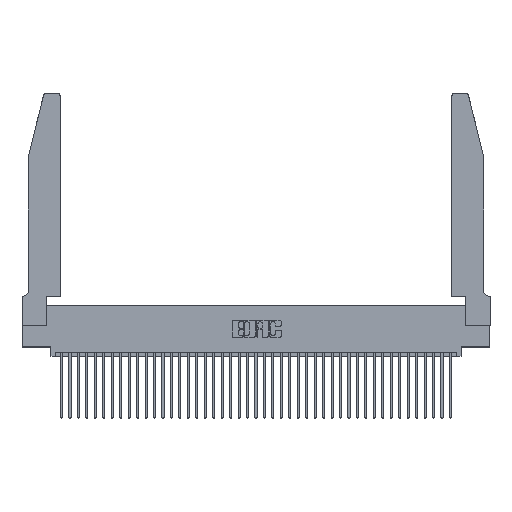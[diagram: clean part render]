
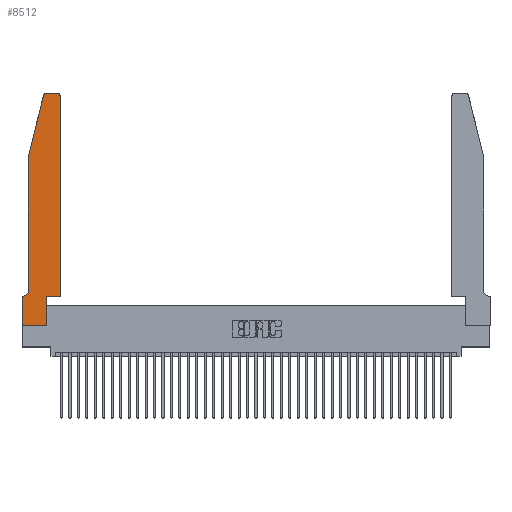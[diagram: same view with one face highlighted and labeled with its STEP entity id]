
A CAD part, top view. The second image highlights one B-rep face of the part: STEP entity #8512.
In plain terms, the highlighted planar face has unit normal (0, 0, 1).
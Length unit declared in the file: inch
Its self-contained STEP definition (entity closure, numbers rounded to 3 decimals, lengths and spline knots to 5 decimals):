
#678 = CARTESIAN_POINT ( 'NONE',  ( 0.0755, 0.35, 0.37 ) ) ;
#826 = CARTESIAN_POINT ( 'NONE',  ( 0.2865, 0.35, 0.37 ) ) ;
#832 = DIRECTION ( 'NONE',  ( 0., 0., -1. ) ) ;
#1188 = CARTESIAN_POINT ( 'NONE',  ( 0., 0., 0.37 ) ) ;
#1258 = CARTESIAN_POINT ( 'NONE',  ( 0.4505, 2.72, 0.37 ) ) ;
#1440 = AXIS2_PLACEMENT_3D ( 'NONE', #15298, #37526, #18527 ) ;
#1489 = VERTEX_POINT ( 'NONE', #26710 ) ;
#1978 = PLANE ( 'NONE',  #31422 ) ;
#2135 = CARTESIAN_POINT ( 'NONE',  ( 0., 0., 0.37 ) ) ;
#2276 = DIRECTION ( 'NONE',  ( -1., 0., 0. ) ) ;
#2727 = CARTESIAN_POINT ( 'NONE',  ( 0.4505, 0.35, 0.37 ) ) ;
#2892 = EDGE_CURVE ( 'NONE', #30835, #19793, #9939, .T. ) ;
#3472 = VERTEX_POINT ( 'NONE', #5498 ) ;
#3788 = ORIENTED_EDGE ( 'NONE', *, *, #40106, .T. ) ;
#4532 = CARTESIAN_POINT ( 'NONE',  ( 0.0755, 2., 0.37 ) ) ;
#5012 = AXIS2_PLACEMENT_3D ( 'NONE', #15292, #37517, #18522 ) ;
#5312 = LINE ( 'NONE', #4532, #30710 ) ;
#5498 = CARTESIAN_POINT ( 'NONE',  ( 0., 0.35, 0.37 ) ) ;
#5663 = DIRECTION ( 'NONE',  ( 0., -1., 0. ) ) ;
#6434 = CARTESIAN_POINT ( 'NONE',  ( 0.0055, 0.35, 0.37 ) ) ;
#6936 = CARTESIAN_POINT ( 'NONE',  ( 0., 0., 0.37 ) ) ;
#8348 = DIRECTION ( 'NONE',  ( 0., 0., 1. ) ) ;
#8512 = ADVANCED_FACE ( 'NONE', ( #18031 ), #1978, .T. ) ;
#8735 = VECTOR ( 'NONE', #26225, 39.37008 ) ;
#9711 = LINE ( 'NONE', #10306, #8735 ) ;
#9939 = LINE ( 'NONE', #2135, #10926 ) ;
#10101 = DIRECTION ( 'NONE',  ( 0., -1., 0. ) ) ;
#10306 = CARTESIAN_POINT ( 'NONE',  ( 0.4505, 0.35, 0.37 ) ) ;
#10403 = CIRCLE ( 'NONE', #15994, 0.07 ) ;
#10580 = EDGE_CURVE ( 'NONE', #26769, #32802, #10403, .T. ) ;
#10926 = VECTOR ( 'NONE', #24395, 39.37008 ) ;
#12018 = CARTESIAN_POINT ( 'NONE',  ( 0.2865, 0., 0.37 ) ) ;
#13012 = ORIENTED_EDGE ( 'NONE', *, *, #10580, .T. ) ;
#13527 = LINE ( 'NONE', #6936, #36921 ) ;
#14370 = ORIENTED_EDGE ( 'NONE', *, *, #40673, .T. ) ;
#14925 = EDGE_CURVE ( 'NONE', #25619, #15075, #20654, .T. ) ;
#15075 = VERTEX_POINT ( 'NONE', #37005 ) ;
#15106 = CARTESIAN_POINT ( 'NONE',  ( 0.0755, 2., 0.37 ) ) ;
#15292 = CARTESIAN_POINT ( 'NONE',  ( 0.284, 2.72, 0.37 ) ) ;
#15298 = CARTESIAN_POINT ( 'NONE',  ( 0.4205, 2.72, 0.37 ) ) ;
#15994 = AXIS2_PLACEMENT_3D ( 'NONE', #19891, #832, #23103 ) ;
#16298 = ORIENTED_EDGE ( 'NONE', *, *, #28432, .T. ) ;
#16540 = DIRECTION ( 'NONE',  ( -1., 0., 0. ) ) ;
#17356 = ORIENTED_EDGE ( 'NONE', *, *, #30061, .T. ) ;
#17877 = LINE ( 'NONE', #32700, #25348 ) ;
#18031 = FACE_OUTER_BOUND ( 'NONE', #25419, .T. ) ;
#18522 = DIRECTION ( 'NONE',  ( 1., 0., 0. ) ) ;
#18527 = DIRECTION ( 'NONE',  ( 1., 0., 0. ) ) ;
#18738 = ORIENTED_EDGE ( 'NONE', *, *, #28729, .T. ) ;
#19155 = LINE ( 'NONE', #678, #26623 ) ;
#19793 = VERTEX_POINT ( 'NONE', #12018 ) ;
#19803 = VECTOR ( 'NONE', #5663, 39.37008 ) ;
#19891 = CARTESIAN_POINT ( 'NONE',  ( 0.0055, 0.42, 0.37 ) ) ;
#20654 = CIRCLE ( 'NONE', #1440, 0.03 ) ;
#20676 = CIRCLE ( 'NONE', #5012, 0.03 ) ;
#20862 = VECTOR ( 'NONE', #2276, 39.37008 ) ;
#21792 = DIRECTION ( 'NONE',  ( 0., 1., 0. ) ) ;
#21812 = LINE ( 'NONE', #15106, #19803 ) ;
#21869 = LINE ( 'NONE', #33970, #20862 ) ;
#23038 = VERTEX_POINT ( 'NONE', #33370 ) ;
#23103 = DIRECTION ( 'NONE',  ( -1., 0., 0. ) ) ;
#23373 = ORIENTED_EDGE ( 'NONE', *, *, #2892, .T. ) ;
#24395 = DIRECTION ( 'NONE',  ( 1., 0., 0. ) ) ;
#25348 = VECTOR ( 'NONE', #35876, 39.37008 ) ;
#25419 = EDGE_LOOP ( 'NONE', ( #36100, #16298, #3788, #39818, #13012, #18738, #17356, #23373, #39348, #14370, #31836, #27286 ) ) ;
#25512 = EDGE_CURVE ( 'NONE', #19793, #30121, #17877, .T. ) ;
#25619 = VERTEX_POINT ( 'NONE', #1258 ) ;
#26225 = DIRECTION ( 'NONE',  ( 1., 0., 0. ) ) ;
#26614 = CARTESIAN_POINT ( 'NONE',  ( 0.25487, 2.72718, 0.37 ) ) ;
#26623 = VECTOR ( 'NONE', #16540, 39.37008 ) ;
#26710 = CARTESIAN_POINT ( 'NONE',  ( 0.4505, 0.35, 0.37 ) ) ;
#26769 = VERTEX_POINT ( 'NONE', #35604 ) ;
#27130 = EDGE_CURVE ( 'NONE', #23038, #26769, #21812, .T. ) ;
#27286 = ORIENTED_EDGE ( 'NONE', *, *, #14925, .T. ) ;
#27428 = CARTESIAN_POINT ( 'NONE',  ( 0., 0.35, 0.37 ) ) ;
#28214 = VECTOR ( 'NONE', #21792, 39.37008 ) ;
#28432 = EDGE_CURVE ( 'NONE', #33786, #38752, #20676, .T. ) ;
#28729 = EDGE_CURVE ( 'NONE', #32802, #3472, #19155, .T. ) ;
#30061 = EDGE_CURVE ( 'NONE', #3472, #30835, #13527, .T. ) ;
#30121 = VERTEX_POINT ( 'NONE', #826 ) ;
#30608 = DIRECTION ( 'NONE',  ( 1., 0., 0. ) ) ;
#30710 = VECTOR ( 'NONE', #39517, 39.37008 ) ;
#30835 = VERTEX_POINT ( 'NONE', #1188 ) ;
#31422 = AXIS2_PLACEMENT_3D ( 'NONE', #27428, #8348, #30608 ) ;
#31836 = ORIENTED_EDGE ( 'NONE', *, *, #40400, .T. ) ;
#32700 = CARTESIAN_POINT ( 'NONE',  ( 0.2865, 0.35, 0.37 ) ) ;
#32802 = VERTEX_POINT ( 'NONE', #6434 ) ;
#33370 = CARTESIAN_POINT ( 'NONE',  ( 0.0755, 2., 0.37 ) ) ;
#33786 = VERTEX_POINT ( 'NONE', #37351 ) ;
#33970 = CARTESIAN_POINT ( 'NONE',  ( 0.2605, 2.75, 0.37 ) ) ;
#35604 = CARTESIAN_POINT ( 'NONE',  ( 0.0755, 0.42, 0.37 ) ) ;
#35654 = LINE ( 'NONE', #2727, #28214 ) ;
#35876 = DIRECTION ( 'NONE',  ( 0., 1., 0. ) ) ;
#36100 = ORIENTED_EDGE ( 'NONE', *, *, #39022, .T. ) ;
#36921 = VECTOR ( 'NONE', #10101, 39.37008 ) ;
#37005 = CARTESIAN_POINT ( 'NONE',  ( 0.4205, 2.75, 0.37 ) ) ;
#37351 = CARTESIAN_POINT ( 'NONE',  ( 0.284, 2.75, 0.37 ) ) ;
#37517 = DIRECTION ( 'NONE',  ( 0., 0., 1. ) ) ;
#37526 = DIRECTION ( 'NONE',  ( 0., 0., 1. ) ) ;
#38752 = VERTEX_POINT ( 'NONE', #26614 ) ;
#39022 = EDGE_CURVE ( 'NONE', #15075, #33786, #21869, .T. ) ;
#39348 = ORIENTED_EDGE ( 'NONE', *, *, #25512, .T. ) ;
#39517 = DIRECTION ( 'NONE',  ( -0.239, -0.971, 0. ) ) ;
#39818 = ORIENTED_EDGE ( 'NONE', *, *, #27130, .T. ) ;
#40106 = EDGE_CURVE ( 'NONE', #38752, #23038, #5312, .T. ) ;
#40400 = EDGE_CURVE ( 'NONE', #1489, #25619, #35654, .T. ) ;
#40673 = EDGE_CURVE ( 'NONE', #30121, #1489, #9711, .T. ) ;
